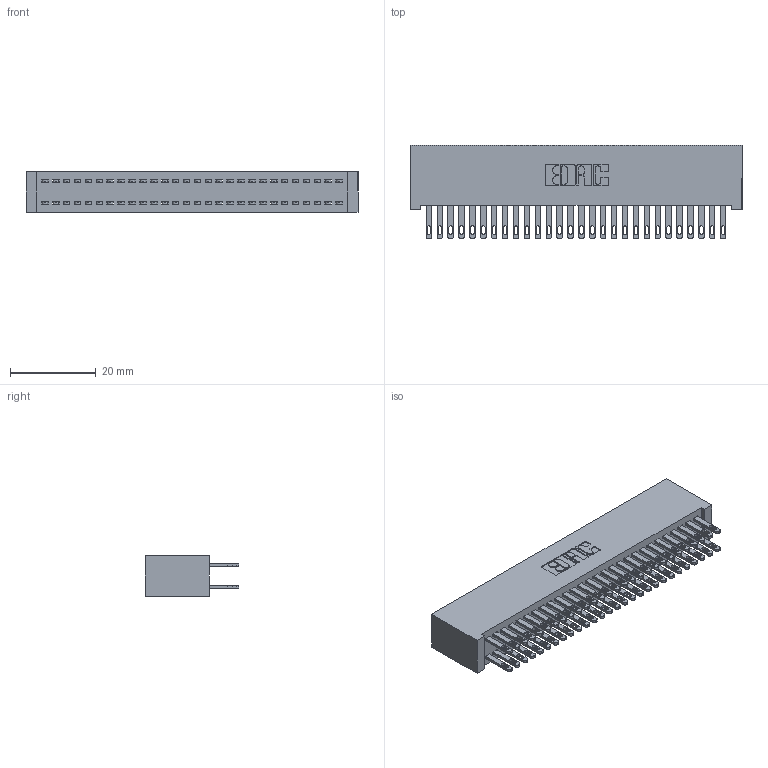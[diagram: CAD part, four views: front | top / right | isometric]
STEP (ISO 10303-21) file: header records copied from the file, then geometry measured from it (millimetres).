
FILE_DESCRIPTION (( 'STEP AP203' ), '1' );
FILE_NAME ('342-056-500-201.STEP', '2018-08-13T02:03:58', ( '' ), ( '' ), 'SwSTEP 2.0', 'SolidWorks 2016', '' );
FILE_SCHEMA (( 'CONFIG_CONTROL_DESIGN' ));
Length unit declared in the file: inch
Products named in the file (3): 342 Part_Lugless; 345-292-001_345-293-100; 342-056-500-201
Assembly tree (57 placements, depth 2):
  342-056-500-201
    342 Part_Lugless
    345-292-001_345-293-100  x56
Bounding box: 77.37 x 21.85 x 9.4 mm (x, y, z)
Volume: 7495.9 mm3; surface area: 12838.9 mm2
Topology: 57 solids, 57 shells, 2790 faces, 8507 edges, 5670 vertices
Faces by surface type: plane 1742, cylinder 1048
Entity records: 19345 total; most frequent: CARTESIAN_POINT 3218, ORIENTED_EDGE 3154, DIRECTION 2769, EDGE_CURVE 1577, LINE 1453, VECTOR 1453, VERTEX_POINT 1050, AXIS2_PLACEMENT_3D 658
